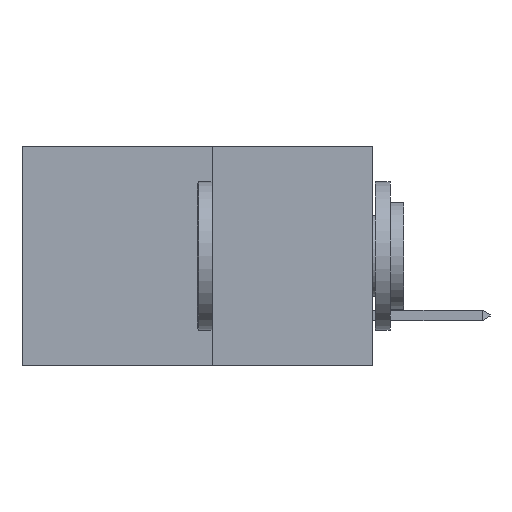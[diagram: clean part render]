
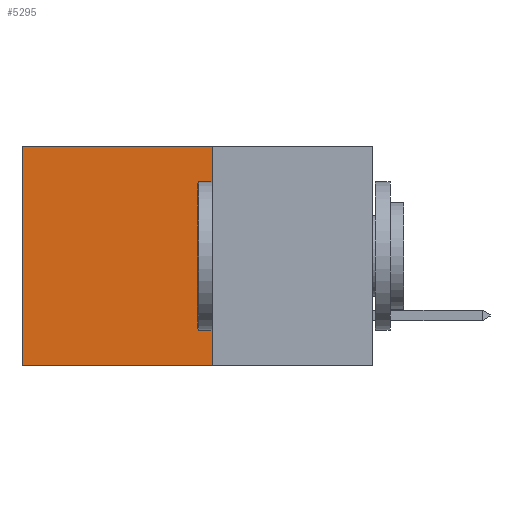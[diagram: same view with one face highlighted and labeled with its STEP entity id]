
A CAD part, left-side view. The second image highlights one B-rep face of the part: STEP entity #5295.
In plain terms, the highlighted planar face has unit normal (-1, 0, 0).
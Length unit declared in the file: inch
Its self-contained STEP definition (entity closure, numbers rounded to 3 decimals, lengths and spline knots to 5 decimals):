
#86 = LINE ( 'NONE', #11108, #9641 ) ;
#362 = VECTOR ( 'NONE', #5542, 39.37008 ) ;
#865 = CARTESIAN_POINT ( 'NONE',  ( 0.277, 0.27, -0.37 ) ) ;
#2316 = EDGE_LOOP ( 'NONE', ( #4953, #5055, #5206, #5264 ) ) ;
#2579 = VERTEX_POINT ( 'NONE', #865 ) ;
#3650 = AXIS2_PLACEMENT_3D ( 'NONE', #8470, #8431, #8414 ) ;
#4107 = EDGE_CURVE ( 'NONE', #11641, #11181, #7477, .T. ) ;
#4248 = DIRECTION ( 'NONE',  ( 0., 0., -1. ) ) ;
#4357 = CARTESIAN_POINT ( 'NONE',  ( 0.277, 0.27, -0.37 ) ) ;
#4441 = FACE_OUTER_BOUND ( 'NONE', #2316, .T. ) ;
#4490 = LINE ( 'NONE', #4357, #9080 ) ;
#4953 = ORIENTED_EDGE ( 'NONE', *, *, #10059, .T. ) ;
#5055 = ORIENTED_EDGE ( 'NONE', *, *, #10502, .F. ) ;
#5206 = ORIENTED_EDGE ( 'NONE', *, *, #9231, .F. ) ;
#5264 = ORIENTED_EDGE ( 'NONE', *, *, #4107, .T. ) ;
#5295 = ADVANCED_FACE ( 'NONE', ( #4441 ), #8859, .F. ) ;
#5542 = DIRECTION ( 'NONE',  ( 0., 1., 0. ) ) ;
#7192 = CARTESIAN_POINT ( 'NONE',  ( 0.277, 0.27, 0. ) ) ;
#7474 = LINE ( 'NONE', #11863, #362 ) ;
#7477 = LINE ( 'NONE', #9004, #9922 ) ;
#7481 = DIRECTION ( 'NONE',  ( 0., 0., -1. ) ) ;
#8405 = VERTEX_POINT ( 'NONE', #11437 ) ;
#8414 = DIRECTION ( 'NONE',  ( 0., 0., -1. ) ) ;
#8431 = DIRECTION ( 'NONE',  ( 1., 0., 0. ) ) ;
#8470 = CARTESIAN_POINT ( 'NONE',  ( 0.277, 0.27, -0.37 ) ) ;
#8859 = PLANE ( 'NONE',  #3650 ) ;
#9004 = CARTESIAN_POINT ( 'NONE',  ( 0.277, 0.27, 0. ) ) ;
#9031 = DIRECTION ( 'NONE',  ( 0., 1., 0. ) ) ;
#9080 = VECTOR ( 'NONE', #4248, 39.37008 ) ;
#9231 = EDGE_CURVE ( 'NONE', #11641, #2579, #4490, .T. ) ;
#9265 = CARTESIAN_POINT ( 'NONE',  ( 0.277, 0.59, 0. ) ) ;
#9641 = VECTOR ( 'NONE', #7481, 39.37008 ) ;
#9922 = VECTOR ( 'NONE', #9031, 39.37008 ) ;
#10059 = EDGE_CURVE ( 'NONE', #11181, #8405, #86, .T. ) ;
#10502 = EDGE_CURVE ( 'NONE', #2579, #8405, #7474, .T. ) ;
#11108 = CARTESIAN_POINT ( 'NONE',  ( 0.277, 0.59, -0.37 ) ) ;
#11181 = VERTEX_POINT ( 'NONE', #9265 ) ;
#11437 = CARTESIAN_POINT ( 'NONE',  ( 0.277, 0.59, -0.37 ) ) ;
#11641 = VERTEX_POINT ( 'NONE', #7192 ) ;
#11863 = CARTESIAN_POINT ( 'NONE',  ( 0.277, 0.27, -0.37 ) ) ;
